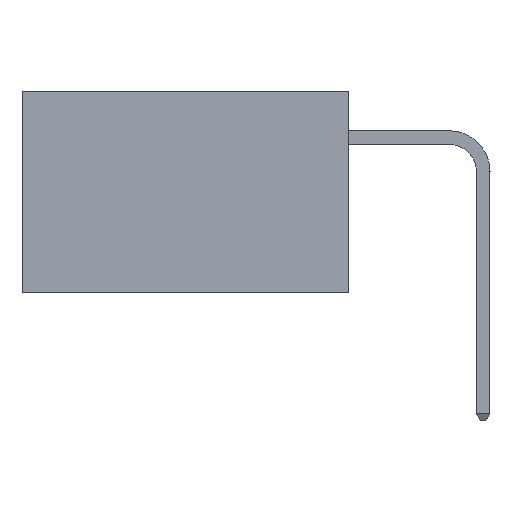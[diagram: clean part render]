
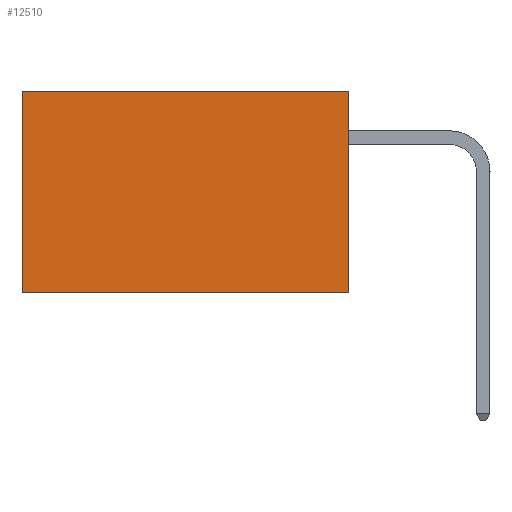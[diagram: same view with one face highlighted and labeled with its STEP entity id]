
A CAD part, left-side view. The second image highlights one B-rep face of the part: STEP entity #12510.
In plain terms, the highlighted planar face has unit normal (-1, 0, 0).
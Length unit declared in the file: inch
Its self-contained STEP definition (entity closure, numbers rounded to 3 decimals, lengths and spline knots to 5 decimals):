
#23 = EDGE_CURVE ( 'NONE', #20607, #11501, #14475, .T. ) ;
#730 = AXIS2_PLACEMENT_3D ( 'NONE', #13552, #1962, #15410 ) ;
#917 = EDGE_LOOP ( 'NONE', ( #13196, #15056, #20007, #5237 ) ) ;
#1962 = DIRECTION ( 'NONE',  ( 1., 0., 0. ) ) ;
#2073 = EDGE_CURVE ( 'NONE', #20607, #19992, #4889, .T. ) ;
#4341 = VECTOR ( 'NONE', #21978, 39.37008 ) ;
#4889 = LINE ( 'NONE', #23433, #23642 ) ;
#5237 = ORIENTED_EDGE ( 'NONE', *, *, #23, .T. ) ;
#7355 = FACE_OUTER_BOUND ( 'NONE', #917, .T. ) ;
#7608 = CARTESIAN_POINT ( 'NONE',  ( 0.2875, 0., 0. ) ) ;
#9717 = CARTESIAN_POINT ( 'NONE',  ( 0.2875, 0., 0. ) ) ;
#9815 = PLANE ( 'NONE',  #730 ) ;
#10698 = DIRECTION ( 'NONE',  ( 0., 1., 0. ) ) ;
#11407 = EDGE_CURVE ( 'NONE', #19992, #14232, #12433, .T. ) ;
#11501 = VERTEX_POINT ( 'NONE', #20079 ) ;
#12433 = LINE ( 'NONE', #21747, #17941 ) ;
#12510 = ADVANCED_FACE ( 'NONE', ( #7355 ), #9815, .F. ) ;
#12951 = LINE ( 'NONE', #24410, #18433 ) ;
#13196 = ORIENTED_EDGE ( 'NONE', *, *, #21112, .T. ) ;
#13552 = CARTESIAN_POINT ( 'NONE',  ( 0.2875, 0., 0. ) ) ;
#14232 = VERTEX_POINT ( 'NONE', #22422 ) ;
#14475 = LINE ( 'NONE', #7608, #4341 ) ;
#15056 = ORIENTED_EDGE ( 'NONE', *, *, #11407, .F. ) ;
#15410 = DIRECTION ( 'NONE',  ( 0., 0., -1. ) ) ;
#15425 = DIRECTION ( 'NONE',  ( 0., 0., -1. ) ) ;
#17051 = DIRECTION ( 'NONE',  ( 0., 0., -1. ) ) ;
#17840 = CARTESIAN_POINT ( 'NONE',  ( 0.2875, 0., -0.37 ) ) ;
#17941 = VECTOR ( 'NONE', #10698, 39.37008 ) ;
#18433 = VECTOR ( 'NONE', #17051, 39.37008 ) ;
#19992 = VERTEX_POINT ( 'NONE', #17840 ) ;
#20007 = ORIENTED_EDGE ( 'NONE', *, *, #2073, .F. ) ;
#20079 = CARTESIAN_POINT ( 'NONE',  ( 0.2875, 0.6, 0. ) ) ;
#20607 = VERTEX_POINT ( 'NONE', #9717 ) ;
#21112 = EDGE_CURVE ( 'NONE', #11501, #14232, #12951, .T. ) ;
#21747 = CARTESIAN_POINT ( 'NONE',  ( 0.2875, 0., -0.37 ) ) ;
#21978 = DIRECTION ( 'NONE',  ( 0., 1., 0. ) ) ;
#22422 = CARTESIAN_POINT ( 'NONE',  ( 0.2875, 0.6, -0.37 ) ) ;
#23433 = CARTESIAN_POINT ( 'NONE',  ( 0.2875, 0., 0. ) ) ;
#23642 = VECTOR ( 'NONE', #15425, 39.37008 ) ;
#24410 = CARTESIAN_POINT ( 'NONE',  ( 0.2875, 0.6, 0. ) ) ;
